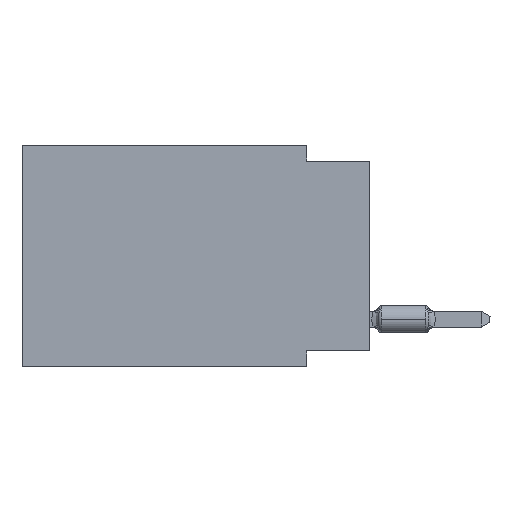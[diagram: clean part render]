
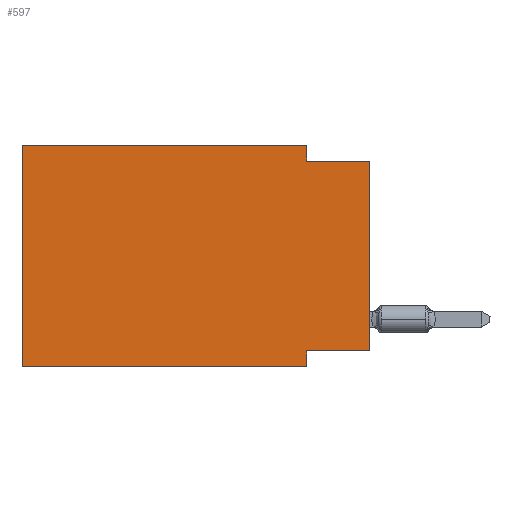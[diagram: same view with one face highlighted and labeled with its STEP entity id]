
A CAD part, left-side view. The second image highlights one B-rep face of the part: STEP entity #597.
In plain terms, the highlighted planar face has unit normal (-1, 0, 0).
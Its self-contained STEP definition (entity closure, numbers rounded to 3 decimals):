
#556 = ORIENTED_EDGE ( 'NONE', *, *, #26227, .F. ) ;
#597 = ADVANCED_FACE ( 'NONE', ( #68255 ), #68665, .F. ) ;
#2496 = DIRECTION ( 'NONE',  ( 0., 0., -1. ) ) ;
#3709 = ORIENTED_EDGE ( 'NONE', *, *, #77001, .T. ) ;
#4768 = VECTOR ( 'NONE', #41970, 1000. ) ;
#4890 = DIRECTION ( 'NONE',  ( 0., -1., 0. ) ) ;
#8174 = VECTOR ( 'NONE', #4890, 1000. ) ;
#8872 = VERTEX_POINT ( 'NONE', #10651 ) ;
#9139 = ORIENTED_EDGE ( 'NONE', *, *, #59752, .T. ) ;
#9268 = DIRECTION ( 'NONE',  ( 0., -1., 0. ) ) ;
#10651 = CARTESIAN_POINT ( 'NONE',  ( 0., 13.97, 0. ) ) ;
#11538 = CARTESIAN_POINT ( 'NONE',  ( 0., 2.54, -0.635 ) ) ;
#12251 = VECTOR ( 'NONE', #2496, 1000. ) ;
#13665 = DIRECTION ( 'NONE',  ( 0., 0., -1. ) ) ;
#14464 = VECTOR ( 'NONE', #74646, 1000. ) ;
#19806 = VECTOR ( 'NONE', #30175, 1000. ) ;
#20149 = CARTESIAN_POINT ( 'NONE',  ( 0., 13.97, -8.89 ) ) ;
#21898 = CARTESIAN_POINT ( 'NONE',  ( 0., 13.97, 0. ) ) ;
#23022 = LINE ( 'NONE', #46474, #40914 ) ;
#23406 = LINE ( 'NONE', #21898, #4768 ) ;
#23876 = ORIENTED_EDGE ( 'NONE', *, *, #58565, .F. ) ;
#23931 = ORIENTED_EDGE ( 'NONE', *, *, #62843, .F. ) ;
#24823 = VERTEX_POINT ( 'NONE', #11538 ) ;
#26227 = EDGE_CURVE ( 'NONE', #24823, #66313, #38982, .T. ) ;
#27036 = ORIENTED_EDGE ( 'NONE', *, *, #71679, .F. ) ;
#28251 = VERTEX_POINT ( 'NONE', #60868 ) ;
#30175 = DIRECTION ( 'NONE',  ( 0., 0., -1. ) ) ;
#31814 = CARTESIAN_POINT ( 'NONE',  ( 0., 0., 0. ) ) ;
#32116 = LINE ( 'NONE', #45803, #35234 ) ;
#33745 = VECTOR ( 'NONE', #51096, 1000. ) ;
#35234 = VECTOR ( 'NONE', #64013, 1000. ) ;
#36051 = CARTESIAN_POINT ( 'NONE',  ( 0., 0., -8.255 ) ) ;
#38238 = ORIENTED_EDGE ( 'NONE', *, *, #58871, .F. ) ;
#38982 = LINE ( 'NONE', #57556, #33745 ) ;
#39201 = AXIS2_PLACEMENT_3D ( 'NONE', #51253, #75129, #13665 ) ;
#39553 = EDGE_LOOP ( 'NONE', ( #3709, #556, #38238, #27036, #23876, #9139, #23931, #79557 ) ) ;
#40914 = VECTOR ( 'NONE', #9268, 1000. ) ;
#41615 = LINE ( 'NONE', #31814, #14464 ) ;
#41970 = DIRECTION ( 'NONE',  ( 0., 0., 1. ) ) ;
#43302 = VERTEX_POINT ( 'NONE', #70025 ) ;
#43926 = VERTEX_POINT ( 'NONE', #20149 ) ;
#45803 = CARTESIAN_POINT ( 'NONE',  ( 0., 0., -8.255 ) ) ;
#46474 = CARTESIAN_POINT ( 'NONE',  ( 0., 13.97, 0. ) ) ;
#51096 = DIRECTION ( 'NONE',  ( 0., -1., 0. ) ) ;
#51253 = CARTESIAN_POINT ( 'NONE',  ( 0., 13.97, 0. ) ) ;
#52875 = VERTEX_POINT ( 'NONE', #36051 ) ;
#54612 = CARTESIAN_POINT ( 'NONE',  ( 0., 13.97, -8.89 ) ) ;
#55786 = CARTESIAN_POINT ( 'NONE',  ( 0., 0., -0.635 ) ) ;
#56731 = CARTESIAN_POINT ( 'NONE',  ( 0., 2.54, -8.255 ) ) ;
#57556 = CARTESIAN_POINT ( 'NONE',  ( 0., 0., -0.635 ) ) ;
#58565 = EDGE_CURVE ( 'NONE', #43926, #8872, #23406, .T. ) ;
#58871 = EDGE_CURVE ( 'NONE', #43302, #24823, #78241, .T. ) ;
#59071 = CARTESIAN_POINT ( 'NONE',  ( 0., 2.54, -8.89 ) ) ;
#59752 = EDGE_CURVE ( 'NONE', #43926, #28251, #79240, .T. ) ;
#60868 = CARTESIAN_POINT ( 'NONE',  ( 0., 2.54, -8.89 ) ) ;
#62843 = EDGE_CURVE ( 'NONE', #75246, #28251, #77654, .T. ) ;
#64013 = DIRECTION ( 'NONE',  ( 0., 1., 0. ) ) ;
#66313 = VERTEX_POINT ( 'NONE', #55786 ) ;
#68255 = FACE_OUTER_BOUND ( 'NONE', #39553, .T. ) ;
#68665 = PLANE ( 'NONE',  #39201 ) ;
#70025 = CARTESIAN_POINT ( 'NONE',  ( 0., 2.54, 0. ) ) ;
#71679 = EDGE_CURVE ( 'NONE', #8872, #43302, #23022, .T. ) ;
#74646 = DIRECTION ( 'NONE',  ( 0., 0., 1. ) ) ;
#75129 = DIRECTION ( 'NONE',  ( 1., 0., 0. ) ) ;
#75246 = VERTEX_POINT ( 'NONE', #56731 ) ;
#77001 = EDGE_CURVE ( 'NONE', #52875, #66313, #41615, .T. ) ;
#77558 = EDGE_CURVE ( 'NONE', #52875, #75246, #32116, .T. ) ;
#77654 = LINE ( 'NONE', #59071, #12251 ) ;
#78241 = LINE ( 'NONE', #79039, #19806 ) ;
#79039 = CARTESIAN_POINT ( 'NONE',  ( 0., 2.54, 0. ) ) ;
#79240 = LINE ( 'NONE', #54612, #8174 ) ;
#79557 = ORIENTED_EDGE ( 'NONE', *, *, #77558, .F. ) ;
